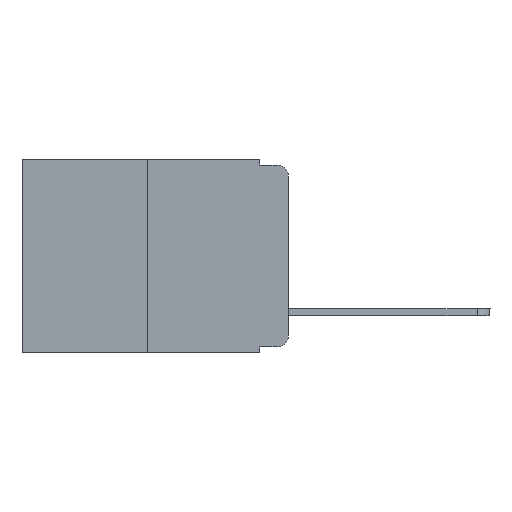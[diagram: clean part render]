
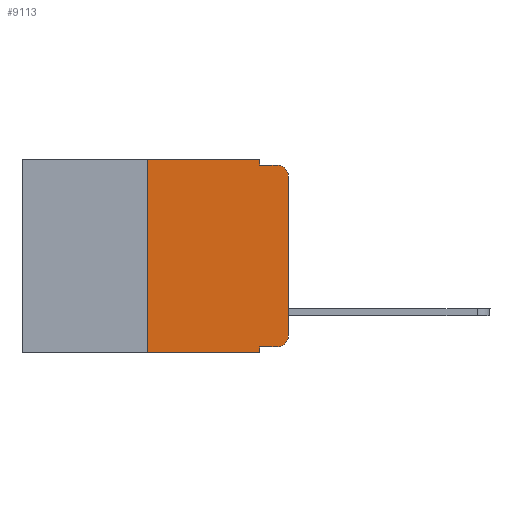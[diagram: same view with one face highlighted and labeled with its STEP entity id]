
A CAD part, left-side view. The second image highlights one B-rep face of the part: STEP entity #9113.
In plain terms, the highlighted planar face has unit normal (-1, 0, 0).
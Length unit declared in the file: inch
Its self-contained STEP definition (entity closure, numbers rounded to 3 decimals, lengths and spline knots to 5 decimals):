
#86 = CARTESIAN_POINT ( 'NONE',  ( 0., 0.25, 0. ) ) ;
#117 = ORIENTED_EDGE ( 'NONE', *, *, #14764, .T. ) ;
#184 = AXIS2_PLACEMENT_3D ( 'NONE', #3955, #24687, #5961 ) ;
#199 = PLANE ( 'NONE',  #184 ) ;
#1343 = LINE ( 'NONE', #21859, #20401 ) ;
#1435 = CARTESIAN_POINT ( 'NONE',  ( 0., 0.051, -0.01 ) ) ;
#2096 = CARTESIAN_POINT ( 'NONE',  ( 0., 0., -0.03 ) ) ;
#2273 = DIRECTION ( 'NONE',  ( 0., 0., -1. ) ) ;
#2660 = AXIS2_PLACEMENT_3D ( 'NONE', #15633, #19646, #2273 ) ;
#2958 = VERTEX_POINT ( 'NONE', #2096 ) ;
#3320 = DIRECTION ( 'NONE',  ( 0., -1., 0. ) ) ;
#3385 = VECTOR ( 'NONE', #23191, 39.37008 ) ;
#3553 = VERTEX_POINT ( 'NONE', #13662 ) ;
#3955 = CARTESIAN_POINT ( 'NONE',  ( 0., 0.473, 0. ) ) ;
#4162 = CIRCLE ( 'NONE', #13322, 0.02 ) ;
#4633 = DIRECTION ( 'NONE',  ( 0., 0., -1. ) ) ;
#4852 = CARTESIAN_POINT ( 'NONE',  ( 0., 0., -0.313 ) ) ;
#5234 = DIRECTION ( 'NONE',  ( 0., -1., 0. ) ) ;
#5476 = ORIENTED_EDGE ( 'NONE', *, *, #19897, .F. ) ;
#5851 = CIRCLE ( 'NONE', #2660, 0.02 ) ;
#5961 = DIRECTION ( 'NONE',  ( 0., 0., -1. ) ) ;
#6015 = LINE ( 'NONE', #15735, #16814 ) ;
#6218 = VERTEX_POINT ( 'NONE', #4852 ) ;
#6496 = LINE ( 'NONE', #14104, #17268 ) ;
#6606 = ORIENTED_EDGE ( 'NONE', *, *, #9173, .F. ) ;
#6912 = CARTESIAN_POINT ( 'NONE',  ( 0., 0.051, 0. ) ) ;
#7306 = EDGE_CURVE ( 'NONE', #9202, #19122, #6496, .T. ) ;
#7608 = ORIENTED_EDGE ( 'NONE', *, *, #9165, .F. ) ;
#7805 = CARTESIAN_POINT ( 'NONE',  ( 0., 0.473, 0. ) ) ;
#9113 = ADVANCED_FACE ( 'NONE', ( #13180 ), #199, .F. ) ;
#9165 = EDGE_CURVE ( 'NONE', #14515, #24141, #9685, .T. ) ;
#9173 = EDGE_CURVE ( 'NONE', #24141, #21086, #15050, .T. ) ;
#9202 = VERTEX_POINT ( 'NONE', #14172 ) ;
#9685 = LINE ( 'NONE', #86, #10936 ) ;
#9870 = DIRECTION ( 'NONE',  ( -1., 0., 0. ) ) ;
#9920 = CARTESIAN_POINT ( 'NONE',  ( 0., 0.02, -0.333 ) ) ;
#10660 = DIRECTION ( 'NONE',  ( 0., 0., -1. ) ) ;
#10768 = ORIENTED_EDGE ( 'NONE', *, *, #11176, .T. ) ;
#10936 = VECTOR ( 'NONE', #11557, 39.37008 ) ;
#11176 = EDGE_CURVE ( 'NONE', #14515, #19122, #6015, .T. ) ;
#11557 = DIRECTION ( 'NONE',  ( 0., 0., 1. ) ) ;
#12221 = ORIENTED_EDGE ( 'NONE', *, *, #14047, .T. ) ;
#13180 = FACE_OUTER_BOUND ( 'NONE', #20135, .T. ) ;
#13213 = CARTESIAN_POINT ( 'NONE',  ( 0., 0.051, -0.343 ) ) ;
#13322 = AXIS2_PLACEMENT_3D ( 'NONE', #15499, #9870, #17497 ) ;
#13413 = CARTESIAN_POINT ( 'NONE',  ( 0., 0., 0. ) ) ;
#13474 = CARTESIAN_POINT ( 'NONE',  ( 0., 0.25, 0. ) ) ;
#13635 = ORIENTED_EDGE ( 'NONE', *, *, #17923, .T. ) ;
#13662 = CARTESIAN_POINT ( 'NONE',  ( 0., 0.02, -0.01 ) ) ;
#14047 = EDGE_CURVE ( 'NONE', #18586, #6218, #4162, .T. ) ;
#14104 = CARTESIAN_POINT ( 'NONE',  ( 0., 0.051, 0. ) ) ;
#14172 = CARTESIAN_POINT ( 'NONE',  ( 0., 0.051, -0.333 ) ) ;
#14515 = VERTEX_POINT ( 'NONE', #20739 ) ;
#14650 = LINE ( 'NONE', #6912, #15116 ) ;
#14764 = EDGE_CURVE ( 'NONE', #6218, #2958, #19317, .T. ) ;
#15050 = LINE ( 'NONE', #7805, #3385 ) ;
#15116 = VECTOR ( 'NONE', #10660, 39.37008 ) ;
#15425 = VECTOR ( 'NONE', #3320, 39.37008 ) ;
#15499 = CARTESIAN_POINT ( 'NONE',  ( 0., 0.02, -0.313 ) ) ;
#15633 = CARTESIAN_POINT ( 'NONE',  ( 0., 0.02, -0.03 ) ) ;
#15680 = CARTESIAN_POINT ( 'NONE',  ( 0., 0.051, 0. ) ) ;
#15735 = CARTESIAN_POINT ( 'NONE',  ( 0., 0.473, -0.343 ) ) ;
#15857 = DIRECTION ( 'NONE',  ( 0., -1., 0. ) ) ;
#16814 = VECTOR ( 'NONE', #15857, 39.37008 ) ;
#17268 = VECTOR ( 'NONE', #4633, 39.37008 ) ;
#17442 = ORIENTED_EDGE ( 'NONE', *, *, #18416, .F. ) ;
#17497 = DIRECTION ( 'NONE',  ( 0., 0., -1. ) ) ;
#17923 = EDGE_CURVE ( 'NONE', #2958, #3553, #5851, .T. ) ;
#18416 = EDGE_CURVE ( 'NONE', #19745, #3553, #23562, .T. ) ;
#18586 = VERTEX_POINT ( 'NONE', #9920 ) ;
#19122 = VERTEX_POINT ( 'NONE', #13213 ) ;
#19317 = LINE ( 'NONE', #13413, #22940 ) ;
#19646 = DIRECTION ( 'NONE',  ( -1., 0., 0. ) ) ;
#19745 = VERTEX_POINT ( 'NONE', #20568 ) ;
#19897 = EDGE_CURVE ( 'NONE', #21086, #19745, #14650, .T. ) ;
#20135 = EDGE_LOOP ( 'NONE', ( #117, #13635, #17442, #5476, #6606, #7608, #10768, #24392, #21079, #12221 ) ) ;
#20401 = VECTOR ( 'NONE', #5234, 39.37008 ) ;
#20568 = CARTESIAN_POINT ( 'NONE',  ( 0., 0.051, -0.01 ) ) ;
#20739 = CARTESIAN_POINT ( 'NONE',  ( 0., 0.25, -0.343 ) ) ;
#21060 = DIRECTION ( 'NONE',  ( 0., 0., 1. ) ) ;
#21079 = ORIENTED_EDGE ( 'NONE', *, *, #24327, .T. ) ;
#21086 = VERTEX_POINT ( 'NONE', #15680 ) ;
#21859 = CARTESIAN_POINT ( 'NONE',  ( 0., 0.051, -0.333 ) ) ;
#22940 = VECTOR ( 'NONE', #21060, 39.37008 ) ;
#23191 = DIRECTION ( 'NONE',  ( 0., -1., 0. ) ) ;
#23562 = LINE ( 'NONE', #1435, #15425 ) ;
#24141 = VERTEX_POINT ( 'NONE', #13474 ) ;
#24327 = EDGE_CURVE ( 'NONE', #9202, #18586, #1343, .T. ) ;
#24392 = ORIENTED_EDGE ( 'NONE', *, *, #7306, .F. ) ;
#24687 = DIRECTION ( 'NONE',  ( 1., 0., 0. ) ) ;
